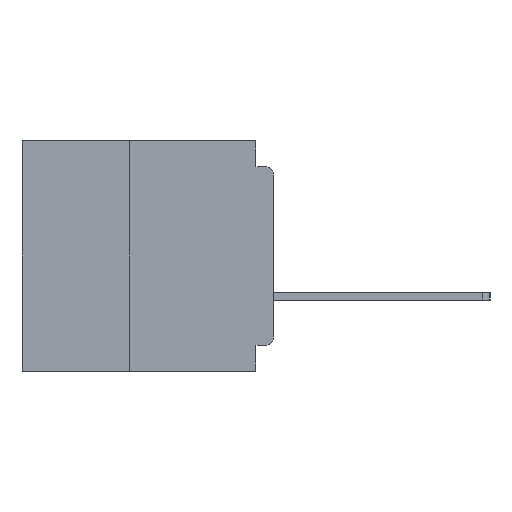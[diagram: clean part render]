
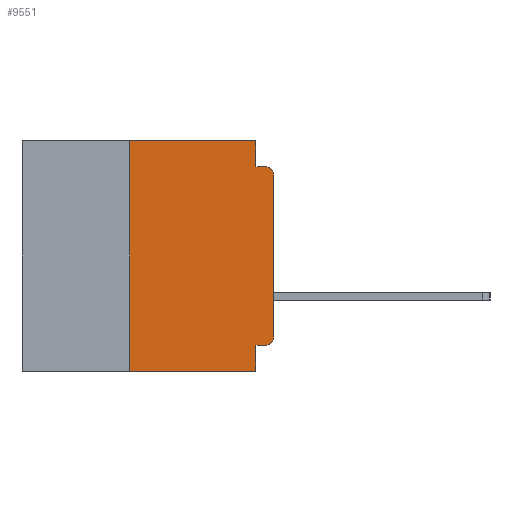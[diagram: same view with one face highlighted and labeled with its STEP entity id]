
A CAD part, left-side view. The second image highlights one B-rep face of the part: STEP entity #9551.
In plain terms, the highlighted planar face has unit normal (-1, 0, 0).
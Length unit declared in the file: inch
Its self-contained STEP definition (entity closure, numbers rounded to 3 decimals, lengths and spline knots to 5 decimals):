
#417 = ORIENTED_EDGE ( 'NONE', *, *, #29183, .F. ) ;
#490 = VECTOR ( 'NONE', #19182, 39.37008 ) ;
#614 = EDGE_CURVE ( 'NONE', #18469, #1120, #1388, .T. ) ;
#1120 = VERTEX_POINT ( 'NONE', #7962 ) ;
#1388 = LINE ( 'NONE', #9183, #490 ) ;
#2132 = ORIENTED_EDGE ( 'NONE', *, *, #10653, .F. ) ;
#2707 = CARTESIAN_POINT ( 'NONE',  ( 0., 0., -0.34 ) ) ;
#3064 = DIRECTION ( 'NONE',  ( -1., 0., 0. ) ) ;
#3370 = DIRECTION ( 'NONE',  ( 0., 0., 1. ) ) ;
#3984 = ORIENTED_EDGE ( 'NONE', *, *, #11220, .F. ) ;
#4737 = VECTOR ( 'NONE', #7346, 39.37008 ) ;
#5134 = VERTEX_POINT ( 'NONE', #6291 ) ;
#5371 = ORIENTED_EDGE ( 'NONE', *, *, #21409, .F. ) ;
#5486 = VECTOR ( 'NONE', #20834, 39.37008 ) ;
#5756 = AXIS2_PLACEMENT_3D ( 'NONE', #12619, #31979, #15442 ) ;
#6097 = VERTEX_POINT ( 'NONE', #13114 ) ;
#6291 = CARTESIAN_POINT ( 'NONE',  ( 0., 0.015, -0.045 ) ) ;
#6839 = CARTESIAN_POINT ( 'NONE',  ( 0., 0.25, -0.4 ) ) ;
#6921 = EDGE_CURVE ( 'NONE', #32958, #14643, #29567, .T. ) ;
#6960 = ORIENTED_EDGE ( 'NONE', *, *, #31266, .T. ) ;
#7072 = CARTESIAN_POINT ( 'NONE',  ( 0., 0.25, 0. ) ) ;
#7108 = PLANE ( 'NONE',  #5756 ) ;
#7346 = DIRECTION ( 'NONE',  ( 0., 0., -1. ) ) ;
#7525 = DIRECTION ( 'NONE',  ( 0., -1., 0. ) ) ;
#7962 = CARTESIAN_POINT ( 'NONE',  ( 0., 0.031, -0.4 ) ) ;
#8440 = ORIENTED_EDGE ( 'NONE', *, *, #35037, .T. ) ;
#9123 = DIRECTION ( 'NONE',  ( 0., 1., 0. ) ) ;
#9183 = CARTESIAN_POINT ( 'NONE',  ( 0., 0.437, -0.4 ) ) ;
#9337 = CARTESIAN_POINT ( 'NONE',  ( 0., 0.031, 0. ) ) ;
#9420 = CARTESIAN_POINT ( 'NONE',  ( 0., 0.031, -0.045 ) ) ;
#9551 = ADVANCED_FACE ( 'NONE', ( #17272 ), #7108, .F. ) ;
#10653 = EDGE_CURVE ( 'NONE', #18469, #18532, #30590, .T. ) ;
#11107 = DIRECTION ( 'NONE',  ( 0., 0., -1. ) ) ;
#11182 = VECTOR ( 'NONE', #3370, 39.37008 ) ;
#11210 = VERTEX_POINT ( 'NONE', #2707 ) ;
#11220 = EDGE_CURVE ( 'NONE', #14643, #1120, #15403, .T. ) ;
#12619 = CARTESIAN_POINT ( 'NONE',  ( 0., 0.437, 0. ) ) ;
#12837 = LINE ( 'NONE', #17996, #5486 ) ;
#13114 = CARTESIAN_POINT ( 'NONE',  ( 0., 0., -0.06 ) ) ;
#13397 = EDGE_LOOP ( 'NONE', ( #8440, #33195, #5371, #417, #18702, #2132, #33752, #3984, #24240, #6960 ) ) ;
#14174 = CARTESIAN_POINT ( 'NONE',  ( 0., 0.015, -0.06 ) ) ;
#14643 = VERTEX_POINT ( 'NONE', #27165 ) ;
#15403 = LINE ( 'NONE', #30479, #21944 ) ;
#15442 = DIRECTION ( 'NONE',  ( 0., 0., -1. ) ) ;
#16974 = DIRECTION ( 'NONE',  ( 0., 0., -1. ) ) ;
#17238 = CARTESIAN_POINT ( 'NONE',  ( 0., 0., 0. ) ) ;
#17272 = FACE_OUTER_BOUND ( 'NONE', #13397, .T. ) ;
#17996 = CARTESIAN_POINT ( 'NONE',  ( 0., 0., -0.045 ) ) ;
#18469 = VERTEX_POINT ( 'NONE', #6839 ) ;
#18532 = VERTEX_POINT ( 'NONE', #7072 ) ;
#18702 = ORIENTED_EDGE ( 'NONE', *, *, #30372, .F. ) ;
#19011 = VERTEX_POINT ( 'NONE', #9337 ) ;
#19094 = CARTESIAN_POINT ( 'NONE',  ( 0., 0.015, -0.355 ) ) ;
#19182 = DIRECTION ( 'NONE',  ( 0., -1., 0. ) ) ;
#19437 = LINE ( 'NONE', #17238, #11182 ) ;
#19737 = CARTESIAN_POINT ( 'NONE',  ( 0., 0.015, -0.34 ) ) ;
#20744 = CIRCLE ( 'NONE', #32500, 0.015 ) ;
#20834 = DIRECTION ( 'NONE',  ( 0., -1., 0. ) ) ;
#21409 = EDGE_CURVE ( 'NONE', #30792, #5134, #12837, .T. ) ;
#21944 = VECTOR ( 'NONE', #11107, 39.37008 ) ;
#22540 = DIRECTION ( 'NONE',  ( 0., 0., -1. ) ) ;
#23107 = VECTOR ( 'NONE', #9123, 39.37008 ) ;
#23939 = CARTESIAN_POINT ( 'NONE',  ( 0., 0.031, 0. ) ) ;
#24240 = ORIENTED_EDGE ( 'NONE', *, *, #6921, .F. ) ;
#25717 = CARTESIAN_POINT ( 'NONE',  ( 0., 0., -0.355 ) ) ;
#26161 = CARTESIAN_POINT ( 'NONE',  ( 0., 0.25, -0.4 ) ) ;
#26988 = CARTESIAN_POINT ( 'NONE',  ( 0., 0.437, 0. ) ) ;
#27165 = CARTESIAN_POINT ( 'NONE',  ( 0., 0.031, -0.355 ) ) ;
#28501 = LINE ( 'NONE', #26988, #35861 ) ;
#28900 = DIRECTION ( 'NONE',  ( 0., 0., 1. ) ) ;
#29183 = EDGE_CURVE ( 'NONE', #19011, #30792, #32465, .T. ) ;
#29247 = AXIS2_PLACEMENT_3D ( 'NONE', #14174, #33556, #16974 ) ;
#29478 = EDGE_CURVE ( 'NONE', #6097, #5134, #32006, .T. ) ;
#29567 = LINE ( 'NONE', #25717, #23107 ) ;
#30372 = EDGE_CURVE ( 'NONE', #18532, #19011, #28501, .T. ) ;
#30479 = CARTESIAN_POINT ( 'NONE',  ( 0., 0.031, -0.4 ) ) ;
#30590 = LINE ( 'NONE', #26161, #34487 ) ;
#30792 = VERTEX_POINT ( 'NONE', #9420 ) ;
#31266 = EDGE_CURVE ( 'NONE', #32958, #11210, #20744, .T. ) ;
#31979 = DIRECTION ( 'NONE',  ( 1., 0., 0. ) ) ;
#32006 = CIRCLE ( 'NONE', #29247, 0.015 ) ;
#32465 = LINE ( 'NONE', #23939, #4737 ) ;
#32500 = AXIS2_PLACEMENT_3D ( 'NONE', #19737, #3064, #22540 ) ;
#32958 = VERTEX_POINT ( 'NONE', #19094 ) ;
#33195 = ORIENTED_EDGE ( 'NONE', *, *, #29478, .T. ) ;
#33556 = DIRECTION ( 'NONE',  ( -1., 0., 0. ) ) ;
#33752 = ORIENTED_EDGE ( 'NONE', *, *, #614, .T. ) ;
#34487 = VECTOR ( 'NONE', #28900, 39.37008 ) ;
#35037 = EDGE_CURVE ( 'NONE', #11210, #6097, #19437, .T. ) ;
#35861 = VECTOR ( 'NONE', #7525, 39.37008 ) ;
